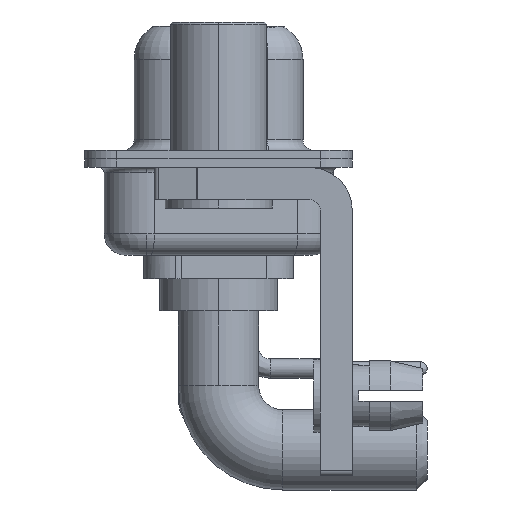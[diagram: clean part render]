
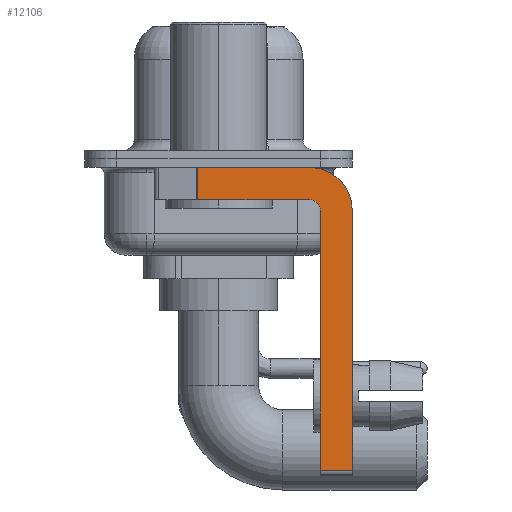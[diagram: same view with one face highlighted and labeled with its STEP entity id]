
A CAD part, left-side view. The second image highlights one B-rep face of the part: STEP entity #12106.
In plain terms, the highlighted planar face has unit normal (-1, 0, 0).
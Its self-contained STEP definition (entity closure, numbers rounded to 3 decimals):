
#496 = AXIS2_PLACEMENT_3D ( 'NONE', #6946, #5312, #3701 ) ;
#601 = DIRECTION ( 'NONE',  ( 0., 0., -1. ) ) ;
#1800 = CARTESIAN_POINT ( 'NONE',  ( -2.9, -4.25, -2.4 ) ) ;
#2007 = DIRECTION ( 'NONE',  ( 1., 0., 0. ) ) ;
#2201 = ORIENTED_EDGE ( 'NONE', *, *, #8534, .F. ) ;
#2428 = EDGE_CURVE ( 'NONE', #6988, #4241, #10862, .T. ) ;
#2492 = EDGE_CURVE ( 'NONE', #12439, #13773, #18578, .T. ) ;
#3691 = ORIENTED_EDGE ( 'NONE', *, *, #9850, .F. ) ;
#3701 = DIRECTION ( 'NONE',  ( 0., 0., 1. ) ) ;
#4241 = VERTEX_POINT ( 'NONE', #10185 ) ;
#4341 = EDGE_CURVE ( 'NONE', #5687, #10464, #9835, .T. ) ;
#5203 = CARTESIAN_POINT ( 'NONE',  ( -2.9, -4.75, -14.55 ) ) ;
#5312 = DIRECTION ( 'NONE',  ( -1., 0., 0. ) ) ;
#5503 = DIRECTION ( 'NONE',  ( 0., 1., 0. ) ) ;
#5549 = ORIENTED_EDGE ( 'NONE', *, *, #16088, .F. ) ;
#5650 = LINE ( 'NONE', #12252, #17405 ) ;
#5687 = VERTEX_POINT ( 'NONE', #13969 ) ;
#6805 = PLANE ( 'NONE',  #17873 ) ;
#6887 = CARTESIAN_POINT ( 'NONE',  ( -2.9, 0.978, -1.9 ) ) ;
#6946 = CARTESIAN_POINT ( 'NONE',  ( -2.9, -4.25, -2.4 ) ) ;
#6988 = VERTEX_POINT ( 'NONE', #15512 ) ;
#7106 = LINE ( 'NONE', #10351, #9660 ) ;
#7405 = AXIS2_PLACEMENT_3D ( 'NONE', #1800, #2007, #8409 ) ;
#8409 = DIRECTION ( 'NONE',  ( 0., 0., -1. ) ) ;
#8534 = EDGE_CURVE ( 'NONE', #14227, #5687, #5650, .T. ) ;
#8919 = VECTOR ( 'NONE', #16989, 1000. ) ;
#9660 = VECTOR ( 'NONE', #17188, 1000. ) ;
#9831 = VECTOR ( 'NONE', #15632, 1000. ) ;
#9835 = CIRCLE ( 'NONE', #496, 0.5 ) ;
#9850 = EDGE_CURVE ( 'NONE', #12439, #6988, #11950, .T. ) ;
#10050 = DIRECTION ( 'NONE',  ( 0., 0., -1. ) ) ;
#10152 = LINE ( 'NONE', #13727, #19597 ) ;
#10185 = CARTESIAN_POINT ( 'NONE',  ( -2.9, -6.25, -2.4 ) ) ;
#10217 = CARTESIAN_POINT ( 'NONE',  ( -2.9, 3., -0.4 ) ) ;
#10351 = CARTESIAN_POINT ( 'NONE',  ( -2.9, -6.25, -2.4 ) ) ;
#10464 = VERTEX_POINT ( 'NONE', #16015 ) ;
#10862 = CIRCLE ( 'NONE', #7405, 2. ) ;
#11050 = ORIENTED_EDGE ( 'NONE', *, *, #2492, .T. ) ;
#11272 = ORIENTED_EDGE ( 'NONE', *, *, #4341, .F. ) ;
#11950 = LINE ( 'NONE', #10217, #9831 ) ;
#12039 = VERTEX_POINT ( 'NONE', #14494 ) ;
#12085 = EDGE_CURVE ( 'NONE', #10464, #13773, #10152, .T. ) ;
#12092 = FACE_OUTER_BOUND ( 'NONE', #14247, .T. ) ;
#12106 = ADVANCED_FACE ( 'NONE', ( #12092 ), #6805, .F. ) ;
#12252 = CARTESIAN_POINT ( 'NONE',  ( -2.9, -4.75, -14.8 ) ) ;
#12368 = CARTESIAN_POINT ( 'NONE',  ( -2.9, 0.978, -1.9 ) ) ;
#12439 = VERTEX_POINT ( 'NONE', #17943 ) ;
#13416 = DIRECTION ( 'NONE',  ( 1., 0., 0. ) ) ;
#13727 = CARTESIAN_POINT ( 'NONE',  ( -2.9, -4.25, -1.9 ) ) ;
#13773 = VERTEX_POINT ( 'NONE', #12368 ) ;
#13969 = CARTESIAN_POINT ( 'NONE',  ( -2.9, -4.75, -2.4 ) ) ;
#14227 = VERTEX_POINT ( 'NONE', #5203 ) ;
#14247 = EDGE_LOOP ( 'NONE', ( #3691, #11050, #17401, #11272, #2201, #19695, #5549, #17093 ) ) ;
#14313 = VECTOR ( 'NONE', #601, 1000. ) ;
#14494 = CARTESIAN_POINT ( 'NONE',  ( -2.9, -6.25, -14.55 ) ) ;
#14612 = EDGE_CURVE ( 'NONE', #14227, #12039, #18711, .T. ) ;
#15466 = CARTESIAN_POINT ( 'NONE',  ( -2.9, -4.25, -2.4 ) ) ;
#15512 = CARTESIAN_POINT ( 'NONE',  ( -2.9, -4.25, -0.4 ) ) ;
#15632 = DIRECTION ( 'NONE',  ( 0., -1., 0. ) ) ;
#16015 = CARTESIAN_POINT ( 'NONE',  ( -2.9, -4.25, -1.9 ) ) ;
#16088 = EDGE_CURVE ( 'NONE', #4241, #12039, #7106, .T. ) ;
#16989 = DIRECTION ( 'NONE',  ( 0., -1., 0. ) ) ;
#17093 = ORIENTED_EDGE ( 'NONE', *, *, #2428, .F. ) ;
#17188 = DIRECTION ( 'NONE',  ( 0., 0., -1. ) ) ;
#17401 = ORIENTED_EDGE ( 'NONE', *, *, #12085, .F. ) ;
#17405 = VECTOR ( 'NONE', #18866, 1000. ) ;
#17873 = AXIS2_PLACEMENT_3D ( 'NONE', #15466, #13416, #10050 ) ;
#17943 = CARTESIAN_POINT ( 'NONE',  ( -2.9, 0.978, -0.4 ) ) ;
#18578 = LINE ( 'NONE', #6887, #14313 ) ;
#18711 = LINE ( 'NONE', #20021, #8919 ) ;
#18866 = DIRECTION ( 'NONE',  ( 0., 0., 1. ) ) ;
#19597 = VECTOR ( 'NONE', #5503, 1000. ) ;
#19695 = ORIENTED_EDGE ( 'NONE', *, *, #14612, .T. ) ;
#20021 = CARTESIAN_POINT ( 'NONE',  ( -2.9, -4.25, -14.55 ) ) ;
